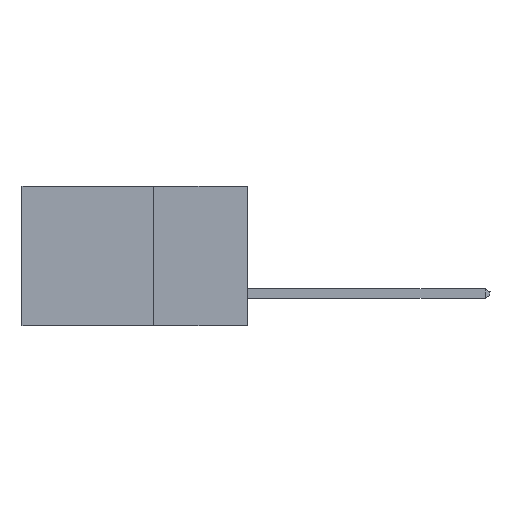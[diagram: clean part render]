
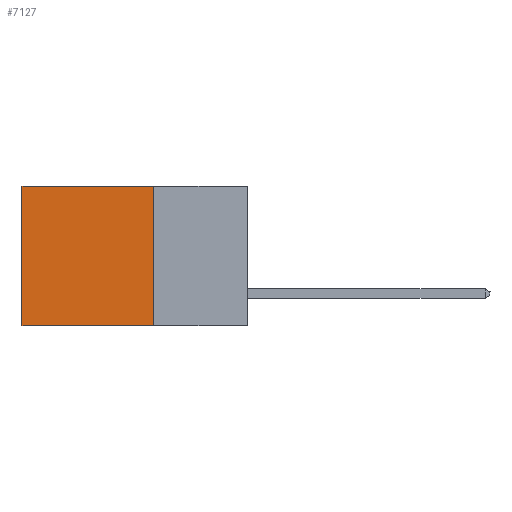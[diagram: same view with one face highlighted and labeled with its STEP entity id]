
A CAD part, left-side view. The second image highlights one B-rep face of the part: STEP entity #7127.
In plain terms, the highlighted planar face has unit normal (-1, 0, 0).
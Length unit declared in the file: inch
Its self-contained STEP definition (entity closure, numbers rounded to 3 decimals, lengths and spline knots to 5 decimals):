
#113 = VECTOR ( 'NONE', #5659, 39.37008 ) ;
#218 = ORIENTED_EDGE ( 'NONE', *, *, #14246, .T. ) ;
#468 = DIRECTION ( 'NONE',  ( 0., 0., -1. ) ) ;
#979 = CARTESIAN_POINT ( 'NONE',  ( 0.2615, 0.25, -0.37 ) ) ;
#1343 = LINE ( 'NONE', #14529, #20861 ) ;
#2234 = VERTEX_POINT ( 'NONE', #20332 ) ;
#2470 = DIRECTION ( 'NONE',  ( 0., 1., 0. ) ) ;
#2691 = DIRECTION ( 'NONE',  ( 0., 0., -1. ) ) ;
#4075 = ORIENTED_EDGE ( 'NONE', *, *, #18736, .T. ) ;
#4444 = EDGE_LOOP ( 'NONE', ( #4075, #14534, #20384, #218 ) ) ;
#5624 = CARTESIAN_POINT ( 'NONE',  ( 0.2615, 0.25, -0.37 ) ) ;
#5659 = DIRECTION ( 'NONE',  ( 0., 1., 0. ) ) ;
#5808 = VECTOR ( 'NONE', #468, 39.37008 ) ;
#6261 = AXIS2_PLACEMENT_3D ( 'NONE', #5624, #10919, #2691 ) ;
#7127 = ADVANCED_FACE ( 'NONE', ( #19156 ), #9087, .F. ) ;
#8803 = CARTESIAN_POINT ( 'NONE',  ( 0.2615, 0.25, -0.37 ) ) ;
#8885 = CARTESIAN_POINT ( 'NONE',  ( 0.2615, 0.6, -0.37 ) ) ;
#9087 = PLANE ( 'NONE',  #6261 ) ;
#9591 = VECTOR ( 'NONE', #10181, 39.37008 ) ;
#10181 = DIRECTION ( 'NONE',  ( 0., 0., -1. ) ) ;
#10919 = DIRECTION ( 'NONE',  ( 1., 0., 0. ) ) ;
#10994 = CARTESIAN_POINT ( 'NONE',  ( 0.2615, 0.6, -0.37 ) ) ;
#11399 = VERTEX_POINT ( 'NONE', #10994 ) ;
#12104 = EDGE_CURVE ( 'NONE', #21378, #11399, #16793, .T. ) ;
#14246 = EDGE_CURVE ( 'NONE', #2234, #20447, #1343, .T. ) ;
#14529 = CARTESIAN_POINT ( 'NONE',  ( 0.2615, 0.25, 0. ) ) ;
#14534 = ORIENTED_EDGE ( 'NONE', *, *, #12104, .F. ) ;
#14947 = LINE ( 'NONE', #16786, #5808 ) ;
#16786 = CARTESIAN_POINT ( 'NONE',  ( 0.2615, 0.25, -0.37 ) ) ;
#16793 = LINE ( 'NONE', #8803, #113 ) ;
#16991 = LINE ( 'NONE', #8885, #9591 ) ;
#18329 = CARTESIAN_POINT ( 'NONE',  ( 0.2615, 0.6, 0. ) ) ;
#18736 = EDGE_CURVE ( 'NONE', #20447, #11399, #16991, .T. ) ;
#19156 = FACE_OUTER_BOUND ( 'NONE', #4444, .T. ) ;
#19473 = EDGE_CURVE ( 'NONE', #2234, #21378, #14947, .T. ) ;
#20332 = CARTESIAN_POINT ( 'NONE',  ( 0.2615, 0.25, 0. ) ) ;
#20384 = ORIENTED_EDGE ( 'NONE', *, *, #19473, .F. ) ;
#20447 = VERTEX_POINT ( 'NONE', #18329 ) ;
#20861 = VECTOR ( 'NONE', #2470, 39.37008 ) ;
#21378 = VERTEX_POINT ( 'NONE', #979 ) ;
